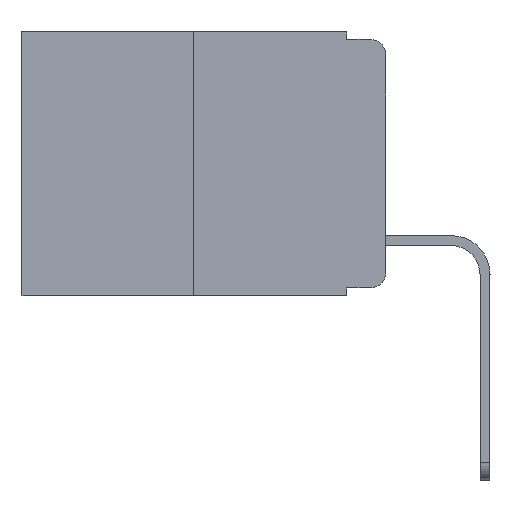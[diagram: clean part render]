
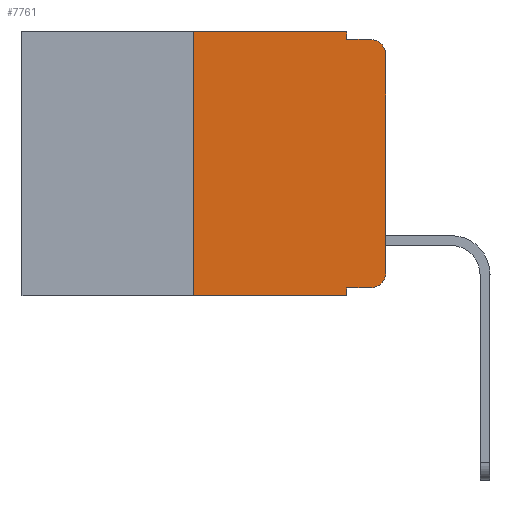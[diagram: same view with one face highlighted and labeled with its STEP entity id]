
A CAD part, left-side view. The second image highlights one B-rep face of the part: STEP entity #7761.
In plain terms, the highlighted planar face has unit normal (-1, 0, 0).
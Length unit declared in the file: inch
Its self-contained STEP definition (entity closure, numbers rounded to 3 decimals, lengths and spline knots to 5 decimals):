
#347 = EDGE_CURVE ( 'NONE', #11937, #12645, #10803, .T. ) ;
#426 = CIRCLE ( 'NONE', #1074, 0.02 ) ;
#440 = DIRECTION ( 'NONE',  ( 0., 0., 1. ) ) ;
#625 = DIRECTION ( 'NONE',  ( 1., 0., 0. ) ) ;
#677 = VECTOR ( 'NONE', #2115, 39.37008 ) ;
#811 = DIRECTION ( 'NONE',  ( 0., 0., -1. ) ) ;
#943 = ORIENTED_EDGE ( 'NONE', *, *, #4658, .F. ) ;
#1074 = AXIS2_PLACEMENT_3D ( 'NONE', #15240, #8746, #11609 ) ;
#1260 = LINE ( 'NONE', #3464, #677 ) ;
#1531 = ORIENTED_EDGE ( 'NONE', *, *, #347, .T. ) ;
#1748 = CARTESIAN_POINT ( 'NONE',  ( 0., 0., -0.03 ) ) ;
#1940 = ORIENTED_EDGE ( 'NONE', *, *, #14502, .T. ) ;
#2103 = VECTOR ( 'NONE', #3691, 39.37008 ) ;
#2115 = DIRECTION ( 'NONE',  ( 0., 0., -1. ) ) ;
#2524 = FACE_OUTER_BOUND ( 'NONE', #11130, .T. ) ;
#2726 = DIRECTION ( 'NONE',  ( 0., 0., -1. ) ) ;
#3215 = DIRECTION ( 'NONE',  ( 0., -1., 0. ) ) ;
#3421 = LINE ( 'NONE', #10098, #11751 ) ;
#3464 = CARTESIAN_POINT ( 'NONE',  ( 0., 0.051, 0. ) ) ;
#3660 = VERTEX_POINT ( 'NONE', #1748 ) ;
#3691 = DIRECTION ( 'NONE',  ( 0., -1., 0. ) ) ;
#3894 = VERTEX_POINT ( 'NONE', #12451 ) ;
#3924 = LINE ( 'NONE', #8940, #2103 ) ;
#4456 = LINE ( 'NONE', #11975, #6079 ) ;
#4658 = EDGE_CURVE ( 'NONE', #12211, #7525, #9492, .T. ) ;
#4683 = CARTESIAN_POINT ( 'NONE',  ( 0., 0.02, -0.313 ) ) ;
#4729 = CARTESIAN_POINT ( 'NONE',  ( 0., 0.473, 0. ) ) ;
#4828 = ORIENTED_EDGE ( 'NONE', *, *, #12886, .F. ) ;
#5396 = CARTESIAN_POINT ( 'NONE',  ( 0., 0.25, -0.343 ) ) ;
#5412 = ORIENTED_EDGE ( 'NONE', *, *, #11961, .F. ) ;
#5504 = VERTEX_POINT ( 'NONE', #6247 ) ;
#5667 = CIRCLE ( 'NONE', #7215, 0.02 ) ;
#5776 = CARTESIAN_POINT ( 'NONE',  ( 0., 0.473, 0. ) ) ;
#5907 = CARTESIAN_POINT ( 'NONE',  ( 0., 0.051, -0.333 ) ) ;
#6048 = VECTOR ( 'NONE', #16738, 39.37008 ) ;
#6079 = VECTOR ( 'NONE', #440, 39.37008 ) ;
#6247 = CARTESIAN_POINT ( 'NONE',  ( 0., 0., -0.313 ) ) ;
#6626 = ORIENTED_EDGE ( 'NONE', *, *, #14691, .T. ) ;
#6951 = CARTESIAN_POINT ( 'NONE',  ( 0., 0.051, -0.333 ) ) ;
#7096 = ORIENTED_EDGE ( 'NONE', *, *, #10756, .T. ) ;
#7215 = AXIS2_PLACEMENT_3D ( 'NONE', #4683, #7284, #811 ) ;
#7284 = DIRECTION ( 'NONE',  ( -1., 0., 0. ) ) ;
#7308 = CARTESIAN_POINT ( 'NONE',  ( 0., 0.02, -0.333 ) ) ;
#7349 = VECTOR ( 'NONE', #3215, 39.37008 ) ;
#7448 = VECTOR ( 'NONE', #15058, 39.37008 ) ;
#7525 = VERTEX_POINT ( 'NONE', #10674 ) ;
#7761 = ADVANCED_FACE ( 'NONE', ( #2524 ), #13523, .F. ) ;
#7980 = CARTESIAN_POINT ( 'NONE',  ( 0., 0.051, 0. ) ) ;
#7984 = ORIENTED_EDGE ( 'NONE', *, *, #8027, .T. ) ;
#8027 = EDGE_CURVE ( 'NONE', #12211, #11604, #3924, .T. ) ;
#8746 = DIRECTION ( 'NONE',  ( -1., 0., 0. ) ) ;
#8940 = CARTESIAN_POINT ( 'NONE',  ( 0., 0.473, -0.343 ) ) ;
#9338 = CARTESIAN_POINT ( 'NONE',  ( 0., 0.02, -0.01 ) ) ;
#9423 = LINE ( 'NONE', #7980, #14661 ) ;
#9492 = LINE ( 'NONE', #14114, #6048 ) ;
#9550 = AXIS2_PLACEMENT_3D ( 'NONE', #5776, #625, #16181 ) ;
#9799 = ORIENTED_EDGE ( 'NONE', *, *, #15167, .F. ) ;
#10098 = CARTESIAN_POINT ( 'NONE',  ( 0., 0.051, -0.01 ) ) ;
#10379 = EDGE_CURVE ( 'NONE', #11937, #11604, #1260, .T. ) ;
#10674 = CARTESIAN_POINT ( 'NONE',  ( 0., 0.25, 0. ) ) ;
#10746 = CARTESIAN_POINT ( 'NONE',  ( 0., 0.051, -0.343 ) ) ;
#10756 = EDGE_CURVE ( 'NONE', #5504, #3660, #4456, .T. ) ;
#10803 = LINE ( 'NONE', #6951, #7349 ) ;
#10804 = VERTEX_POINT ( 'NONE', #13353 ) ;
#11130 = EDGE_LOOP ( 'NONE', ( #7096, #6626, #9799, #4828, #5412, #943, #7984, #11324, #1531, #1940 ) ) ;
#11324 = ORIENTED_EDGE ( 'NONE', *, *, #10379, .F. ) ;
#11604 = VERTEX_POINT ( 'NONE', #10746 ) ;
#11609 = DIRECTION ( 'NONE',  ( 0., 0., -1. ) ) ;
#11751 = VECTOR ( 'NONE', #15159, 39.37008 ) ;
#11937 = VERTEX_POINT ( 'NONE', #5907 ) ;
#11961 = EDGE_CURVE ( 'NONE', #7525, #3894, #16759, .T. ) ;
#11975 = CARTESIAN_POINT ( 'NONE',  ( 0., 0., 0. ) ) ;
#12211 = VERTEX_POINT ( 'NONE', #5396 ) ;
#12451 = CARTESIAN_POINT ( 'NONE',  ( 0., 0.051, 0. ) ) ;
#12645 = VERTEX_POINT ( 'NONE', #7308 ) ;
#12886 = EDGE_CURVE ( 'NONE', #3894, #10804, #9423, .T. ) ;
#12895 = VERTEX_POINT ( 'NONE', #9338 ) ;
#13353 = CARTESIAN_POINT ( 'NONE',  ( 0., 0.051, -0.01 ) ) ;
#13523 = PLANE ( 'NONE',  #9550 ) ;
#14114 = CARTESIAN_POINT ( 'NONE',  ( 0., 0.25, 0. ) ) ;
#14502 = EDGE_CURVE ( 'NONE', #12645, #5504, #5667, .T. ) ;
#14661 = VECTOR ( 'NONE', #2726, 39.37008 ) ;
#14691 = EDGE_CURVE ( 'NONE', #3660, #12895, #426, .T. ) ;
#15058 = DIRECTION ( 'NONE',  ( 0., -1., 0. ) ) ;
#15159 = DIRECTION ( 'NONE',  ( 0., -1., 0. ) ) ;
#15167 = EDGE_CURVE ( 'NONE', #10804, #12895, #3421, .T. ) ;
#15240 = CARTESIAN_POINT ( 'NONE',  ( 0., 0.02, -0.03 ) ) ;
#16181 = DIRECTION ( 'NONE',  ( 0., 0., -1. ) ) ;
#16738 = DIRECTION ( 'NONE',  ( 0., 0., 1. ) ) ;
#16759 = LINE ( 'NONE', #4729, #7448 ) ;
